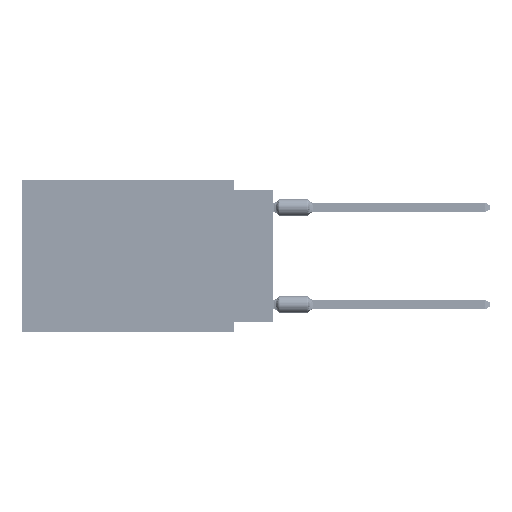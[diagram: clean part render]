
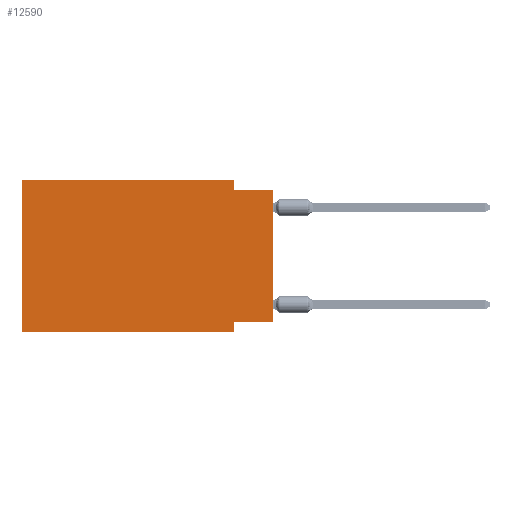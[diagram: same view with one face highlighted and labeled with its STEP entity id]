
A CAD part, left-side view. The second image highlights one B-rep face of the part: STEP entity #12590.
In plain terms, the highlighted planar face has unit normal (-1, 0, 0).
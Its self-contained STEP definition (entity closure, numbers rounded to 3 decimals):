
#1121 = CARTESIAN_POINT ( 'NONE',  ( 0., 0., -9.271 ) ) ;
#3946 = CARTESIAN_POINT ( 'NONE',  ( 0., 16.383, 0. ) ) ;
#4031 = CARTESIAN_POINT ( 'NONE',  ( 0., 0., 0. ) ) ;
#5746 = CARTESIAN_POINT ( 'NONE',  ( 0., 16.383, 0. ) ) ;
#8186 = VECTOR ( 'NONE', #9881, 1000. ) ;
#8801 = LINE ( 'NONE', #52683, #36384 ) ;
#8886 = CARTESIAN_POINT ( 'NONE',  ( 0., 0., -0.635 ) ) ;
#9628 = EDGE_CURVE ( 'NONE', #13756, #70036, #48700, .T. ) ;
#9881 = DIRECTION ( 'NONE',  ( 0., -1., 0. ) ) ;
#9950 = EDGE_CURVE ( 'NONE', #73739, #53568, #60387, .T. ) ;
#10730 = PLANE ( 'NONE',  #40529 ) ;
#10969 = ORIENTED_EDGE ( 'NONE', *, *, #9628, .T. ) ;
#11001 = CARTESIAN_POINT ( 'NONE',  ( 0., 16.383, -9.906 ) ) ;
#11059 = CARTESIAN_POINT ( 'NONE',  ( 0., 16.383, 0. ) ) ;
#12590 = ADVANCED_FACE ( 'NONE', ( #35143 ), #10730, .F. ) ;
#13756 = VERTEX_POINT ( 'NONE', #1121 ) ;
#13999 = DIRECTION ( 'NONE',  ( 0., -1., 0. ) ) ;
#14473 = CARTESIAN_POINT ( 'NONE',  ( 0., 2.54, -9.271 ) ) ;
#16752 = VERTEX_POINT ( 'NONE', #37019 ) ;
#19873 = ORIENTED_EDGE ( 'NONE', *, *, #50878, .F. ) ;
#20285 = CARTESIAN_POINT ( 'NONE',  ( 0., 2.54, 0. ) ) ;
#22644 = DIRECTION ( 'NONE',  ( 0., 0., 1. ) ) ;
#23706 = EDGE_CURVE ( 'NONE', #13756, #45874, #8801, .T. ) ;
#23710 = DIRECTION ( 'NONE',  ( 0., 0., -1. ) ) ;
#24072 = DIRECTION ( 'NONE',  ( 0., -1., 0. ) ) ;
#26589 = CARTESIAN_POINT ( 'NONE',  ( 0., 0., -0.635 ) ) ;
#28633 = DIRECTION ( 'NONE',  ( 1., 0., 0. ) ) ;
#28828 = DIRECTION ( 'NONE',  ( 0., 0., 1. ) ) ;
#29841 = ORIENTED_EDGE ( 'NONE', *, *, #23706, .F. ) ;
#31693 = LINE ( 'NONE', #20285, #59498 ) ;
#32491 = DIRECTION ( 'NONE',  ( 0., 0., -1. ) ) ;
#34075 = EDGE_CURVE ( 'NONE', #73739, #49255, #54561, .T. ) ;
#35143 = FACE_OUTER_BOUND ( 'NONE', #57026, .T. ) ;
#35411 = VECTOR ( 'NONE', #13999, 1000. ) ;
#36384 = VECTOR ( 'NONE', #65623, 1000. ) ;
#37019 = CARTESIAN_POINT ( 'NONE',  ( 0., 2.54, -0.635 ) ) ;
#38744 = EDGE_CURVE ( 'NONE', #16752, #70036, #57449, .T. ) ;
#40529 = AXIS2_PLACEMENT_3D ( 'NONE', #60267, #28633, #59870 ) ;
#41265 = VERTEX_POINT ( 'NONE', #52131 ) ;
#43297 = VECTOR ( 'NONE', #28828, 1000. ) ;
#44477 = EDGE_CURVE ( 'NONE', #41265, #16752, #31693, .T. ) ;
#44478 = VECTOR ( 'NONE', #22644, 1000. ) ;
#45315 = VECTOR ( 'NONE', #24072, 1000. ) ;
#45874 = VERTEX_POINT ( 'NONE', #14473 ) ;
#47694 = CARTESIAN_POINT ( 'NONE',  ( 0., 2.54, -9.906 ) ) ;
#48700 = LINE ( 'NONE', #4031, #43297 ) ;
#49255 = VERTEX_POINT ( 'NONE', #61399 ) ;
#49321 = ORIENTED_EDGE ( 'NONE', *, *, #34075, .T. ) ;
#50878 = EDGE_CURVE ( 'NONE', #53568, #41265, #65479, .T. ) ;
#51291 = EDGE_CURVE ( 'NONE', #45874, #49255, #59052, .T. ) ;
#52131 = CARTESIAN_POINT ( 'NONE',  ( 0., 2.54, 0. ) ) ;
#52683 = CARTESIAN_POINT ( 'NONE',  ( 0., 0., -9.271 ) ) ;
#53568 = VERTEX_POINT ( 'NONE', #5746 ) ;
#54561 = LINE ( 'NONE', #74351, #45315 ) ;
#56971 = ORIENTED_EDGE ( 'NONE', *, *, #44477, .F. ) ;
#57026 = EDGE_LOOP ( 'NONE', ( #10969, #59119, #56971, #19873, #58153, #49321, #59385, #29841 ) ) ;
#57449 = LINE ( 'NONE', #26589, #35411 ) ;
#58153 = ORIENTED_EDGE ( 'NONE', *, *, #9950, .F. ) ;
#59052 = LINE ( 'NONE', #47694, #78263 ) ;
#59119 = ORIENTED_EDGE ( 'NONE', *, *, #38744, .F. ) ;
#59385 = ORIENTED_EDGE ( 'NONE', *, *, #51291, .F. ) ;
#59498 = VECTOR ( 'NONE', #32491, 1000. ) ;
#59870 = DIRECTION ( 'NONE',  ( 0., 0., -1. ) ) ;
#60267 = CARTESIAN_POINT ( 'NONE',  ( 0., 16.383, 0. ) ) ;
#60387 = LINE ( 'NONE', #3946, #44478 ) ;
#61399 = CARTESIAN_POINT ( 'NONE',  ( 0., 2.54, -9.906 ) ) ;
#65479 = LINE ( 'NONE', #11059, #8186 ) ;
#65623 = DIRECTION ( 'NONE',  ( 0., 1., 0. ) ) ;
#70036 = VERTEX_POINT ( 'NONE', #8886 ) ;
#73739 = VERTEX_POINT ( 'NONE', #11001 ) ;
#74351 = CARTESIAN_POINT ( 'NONE',  ( 0., 16.383, -9.906 ) ) ;
#78263 = VECTOR ( 'NONE', #23710, 1000. ) ;
